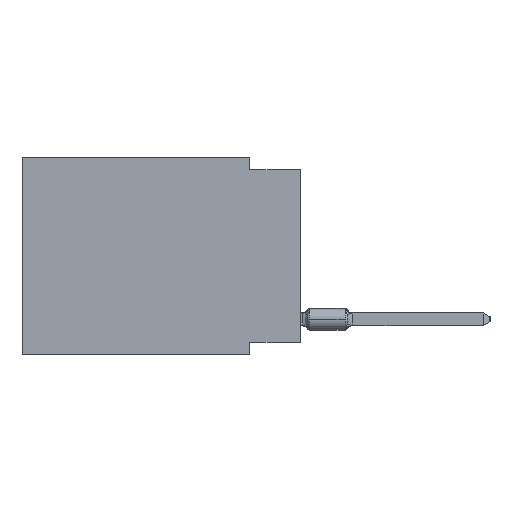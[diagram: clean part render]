
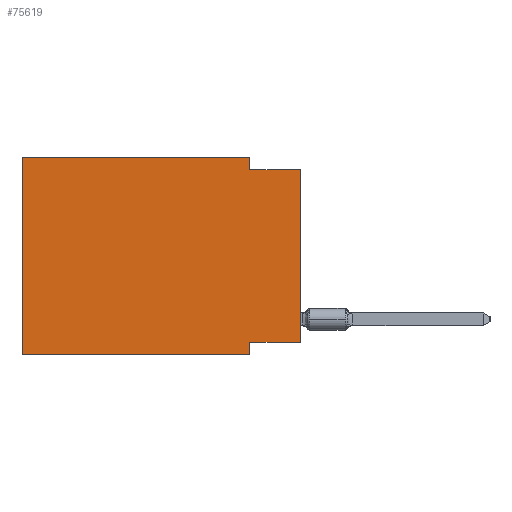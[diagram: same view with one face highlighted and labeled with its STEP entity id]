
A CAD part, left-side view. The second image highlights one B-rep face of the part: STEP entity #75619.
In plain terms, the highlighted planar face has unit normal (-1, 0, 0).
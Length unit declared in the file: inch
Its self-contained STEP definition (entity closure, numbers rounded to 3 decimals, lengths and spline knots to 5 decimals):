
#3319 = CARTESIAN_POINT ( 'NONE',  ( 0., 0.55, -0.39 ) ) ;
#4130 = LINE ( 'NONE', #42545, #22863 ) ;
#7729 = DIRECTION ( 'NONE',  ( 1., 0., 0. ) ) ;
#8967 = FACE_OUTER_BOUND ( 'NONE', #27760, .T. ) ;
#9745 = ORIENTED_EDGE ( 'NONE', *, *, #14867, .F. ) ;
#11110 = CARTESIAN_POINT ( 'NONE',  ( 0., 0.1, 0. ) ) ;
#11670 = EDGE_CURVE ( 'NONE', #71035, #39392, #4130, .T. ) ;
#12575 = CARTESIAN_POINT ( 'NONE',  ( 0., 0.1, -0.365 ) ) ;
#12856 = VERTEX_POINT ( 'NONE', #57963 ) ;
#13505 = ORIENTED_EDGE ( 'NONE', *, *, #11670, .F. ) ;
#14867 = EDGE_CURVE ( 'NONE', #39392, #20598, #64041, .T. ) ;
#16274 = EDGE_CURVE ( 'NONE', #50346, #21135, #51969, .T. ) ;
#20598 = VERTEX_POINT ( 'NONE', #46352 ) ;
#21135 = VERTEX_POINT ( 'NONE', #71546 ) ;
#21451 = DIRECTION ( 'NONE',  ( 0., -1., 0. ) ) ;
#22863 = VECTOR ( 'NONE', #35446, 39.37008 ) ;
#23186 = VECTOR ( 'NONE', #75514, 39.37008 ) ;
#27347 = PLANE ( 'NONE',  #38077 ) ;
#27760 = EDGE_LOOP ( 'NONE', ( #59585, #74794, #41794, #73655, #36034, #30359, #9745, #13505 ) ) ;
#28777 = DIRECTION ( 'NONE',  ( 0., -1., 0. ) ) ;
#29834 = EDGE_CURVE ( 'NONE', #21135, #12856, #80923, .T. ) ;
#30359 = ORIENTED_EDGE ( 'NONE', *, *, #51030, .T. ) ;
#32390 = CARTESIAN_POINT ( 'NONE',  ( 0., 0., -0.025 ) ) ;
#35056 = LINE ( 'NONE', #3319, #81082 ) ;
#35446 = DIRECTION ( 'NONE',  ( 0., 1., 0. ) ) ;
#36034 = ORIENTED_EDGE ( 'NONE', *, *, #67142, .F. ) ;
#37298 = CARTESIAN_POINT ( 'NONE',  ( 0., 0., 0. ) ) ;
#38077 = AXIS2_PLACEMENT_3D ( 'NONE', #47007, #7729, #58717 ) ;
#38947 = DIRECTION ( 'NONE',  ( 0., 0., -1. ) ) ;
#39392 = VERTEX_POINT ( 'NONE', #12575 ) ;
#41794 = ORIENTED_EDGE ( 'NONE', *, *, #29834, .F. ) ;
#42475 = CARTESIAN_POINT ( 'NONE',  ( 0., 0.55, -0.39 ) ) ;
#42545 = CARTESIAN_POINT ( 'NONE',  ( 0., 0., -0.365 ) ) ;
#43205 = LINE ( 'NONE', #37298, #57140 ) ;
#43302 = EDGE_CURVE ( 'NONE', #12856, #59792, #82578, .T. ) ;
#46066 = CARTESIAN_POINT ( 'NONE',  ( 0., 0.1, -0.39 ) ) ;
#46141 = CARTESIAN_POINT ( 'NONE',  ( 0., 0.55, 0. ) ) ;
#46352 = CARTESIAN_POINT ( 'NONE',  ( 0., 0.1, -0.39 ) ) ;
#47007 = CARTESIAN_POINT ( 'NONE',  ( 0., 0.55, 0. ) ) ;
#47417 = LINE ( 'NONE', #79598, #53506 ) ;
#48582 = VECTOR ( 'NONE', #38947, 39.37008 ) ;
#50004 = CARTESIAN_POINT ( 'NONE',  ( 0., 0., -0.025 ) ) ;
#50346 = VERTEX_POINT ( 'NONE', #81216 ) ;
#51030 = EDGE_CURVE ( 'NONE', #57039, #20598, #35056, .T. ) ;
#51635 = EDGE_CURVE ( 'NONE', #71035, #59792, #43205, .T. ) ;
#51969 = LINE ( 'NONE', #46141, #69886 ) ;
#53506 = VECTOR ( 'NONE', #66623, 39.37008 ) ;
#54693 = VECTOR ( 'NONE', #75070, 39.37008 ) ;
#57039 = VERTEX_POINT ( 'NONE', #42475 ) ;
#57140 = VECTOR ( 'NONE', #69101, 39.37008 ) ;
#57963 = CARTESIAN_POINT ( 'NONE',  ( 0., 0.1, -0.025 ) ) ;
#58717 = DIRECTION ( 'NONE',  ( 0., 0., -1. ) ) ;
#59585 = ORIENTED_EDGE ( 'NONE', *, *, #51635, .T. ) ;
#59792 = VERTEX_POINT ( 'NONE', #32390 ) ;
#62204 = CARTESIAN_POINT ( 'NONE',  ( 0., 0., -0.365 ) ) ;
#64041 = LINE ( 'NONE', #46066, #48582 ) ;
#66623 = DIRECTION ( 'NONE',  ( 0., 0., 1. ) ) ;
#67142 = EDGE_CURVE ( 'NONE', #57039, #50346, #47417, .T. ) ;
#69101 = DIRECTION ( 'NONE',  ( 0., 0., 1. ) ) ;
#69886 = VECTOR ( 'NONE', #21451, 39.37008 ) ;
#71035 = VERTEX_POINT ( 'NONE', #62204 ) ;
#71546 = CARTESIAN_POINT ( 'NONE',  ( 0., 0.1, 0. ) ) ;
#73655 = ORIENTED_EDGE ( 'NONE', *, *, #16274, .F. ) ;
#74794 = ORIENTED_EDGE ( 'NONE', *, *, #43302, .F. ) ;
#75070 = DIRECTION ( 'NONE',  ( 0., 0., -1. ) ) ;
#75514 = DIRECTION ( 'NONE',  ( 0., -1., 0. ) ) ;
#75619 = ADVANCED_FACE ( 'NONE', ( #8967 ), #27347, .F. ) ;
#79598 = CARTESIAN_POINT ( 'NONE',  ( 0., 0.55, 0. ) ) ;
#80923 = LINE ( 'NONE', #11110, #54693 ) ;
#81082 = VECTOR ( 'NONE', #28777, 39.37008 ) ;
#81216 = CARTESIAN_POINT ( 'NONE',  ( 0., 0.55, 0. ) ) ;
#82578 = LINE ( 'NONE', #50004, #23186 ) ;
